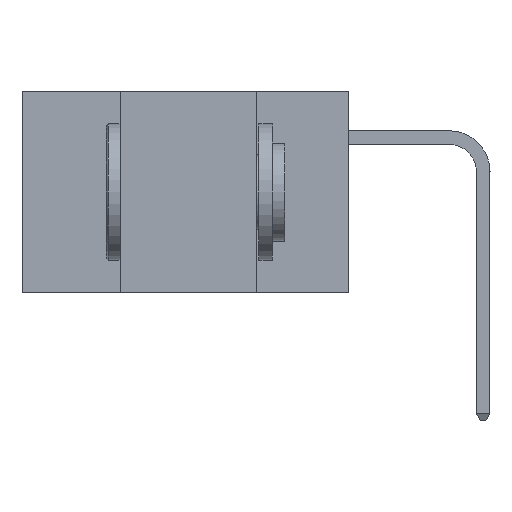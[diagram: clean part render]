
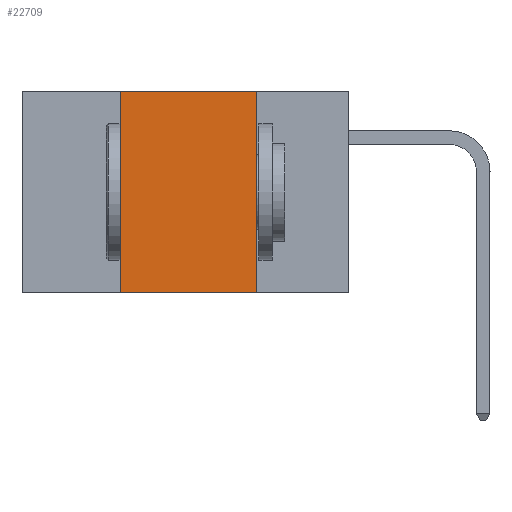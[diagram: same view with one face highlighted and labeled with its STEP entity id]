
A CAD part, left-side view. The second image highlights one B-rep face of the part: STEP entity #22709.
In plain terms, the highlighted planar face has unit normal (-1, 0, 0).
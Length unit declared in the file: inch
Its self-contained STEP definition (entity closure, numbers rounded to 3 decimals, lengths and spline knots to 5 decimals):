
#367 = AXIS2_PLACEMENT_3D ( 'NONE', #24056, #29983, #12395 ) ;
#1588 = VECTOR ( 'NONE', #12167, 39.37008 ) ;
#3983 = EDGE_CURVE ( 'NONE', #20194, #25512, #22024, .T. ) ;
#5991 = ORIENTED_EDGE ( 'NONE', *, *, #33832, .F. ) ;
#8635 = DIRECTION ( 'NONE',  ( 0., 0., -1. ) ) ;
#9399 = PLANE ( 'NONE',  #367 ) ;
#9416 = VERTEX_POINT ( 'NONE', #14711 ) ;
#9673 = ORIENTED_EDGE ( 'NONE', *, *, #13137, .F. ) ;
#10993 = FACE_OUTER_BOUND ( 'NONE', #34761, .T. ) ;
#11564 = ORIENTED_EDGE ( 'NONE', *, *, #3983, .T. ) ;
#12167 = DIRECTION ( 'NONE',  ( 0., 0., 1. ) ) ;
#12395 = DIRECTION ( 'NONE',  ( 0., 0., -1. ) ) ;
#13137 = EDGE_CURVE ( 'NONE', #20194, #9416, #18159, .T. ) ;
#14014 = CARTESIAN_POINT ( 'NONE',  ( 0., 0.17, -0.37 ) ) ;
#14711 = CARTESIAN_POINT ( 'NONE',  ( 0., 0.42, 0. ) ) ;
#14850 = DIRECTION ( 'NONE',  ( 0., -1., 0. ) ) ;
#16894 = CARTESIAN_POINT ( 'NONE',  ( 0., 0.42, -0.37 ) ) ;
#18159 = LINE ( 'NONE', #26676, #1588 ) ;
#19052 = CARTESIAN_POINT ( 'NONE',  ( 0., 0.6, -0.37 ) ) ;
#20194 = VERTEX_POINT ( 'NONE', #16894 ) ;
#20341 = VECTOR ( 'NONE', #14850, 39.37008 ) ;
#21016 = VERTEX_POINT ( 'NONE', #32886 ) ;
#22024 = LINE ( 'NONE', #19052, #29859 ) ;
#22709 = ADVANCED_FACE ( 'NONE', ( #10993 ), #9399, .F. ) ;
#24056 = CARTESIAN_POINT ( 'NONE',  ( 0., 0.6, 0. ) ) ;
#25415 = VECTOR ( 'NONE', #8635, 39.37008 ) ;
#25512 = VERTEX_POINT ( 'NONE', #14014 ) ;
#26544 = CARTESIAN_POINT ( 'NONE',  ( 0., 0.6, 0. ) ) ;
#26676 = CARTESIAN_POINT ( 'NONE',  ( 0., 0.42, 0. ) ) ;
#27791 = EDGE_CURVE ( 'NONE', #21016, #25512, #34105, .T. ) ;
#28158 = LINE ( 'NONE', #26544, #20341 ) ;
#29859 = VECTOR ( 'NONE', #33780, 39.37008 ) ;
#29983 = DIRECTION ( 'NONE',  ( 1., 0., 0. ) ) ;
#30780 = ORIENTED_EDGE ( 'NONE', *, *, #27791, .F. ) ;
#32886 = CARTESIAN_POINT ( 'NONE',  ( 0., 0.17, 0. ) ) ;
#33780 = DIRECTION ( 'NONE',  ( 0., -1., 0. ) ) ;
#33832 = EDGE_CURVE ( 'NONE', #9416, #21016, #28158, .T. ) ;
#34105 = LINE ( 'NONE', #37863, #25415 ) ;
#34761 = EDGE_LOOP ( 'NONE', ( #30780, #5991, #9673, #11564 ) ) ;
#37863 = CARTESIAN_POINT ( 'NONE',  ( 0., 0.17, 0. ) ) ;
